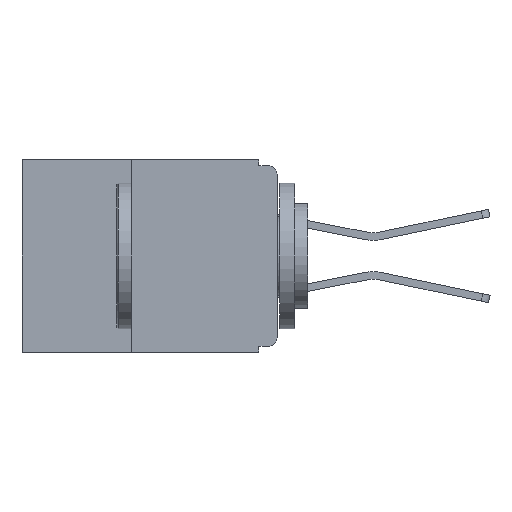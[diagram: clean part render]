
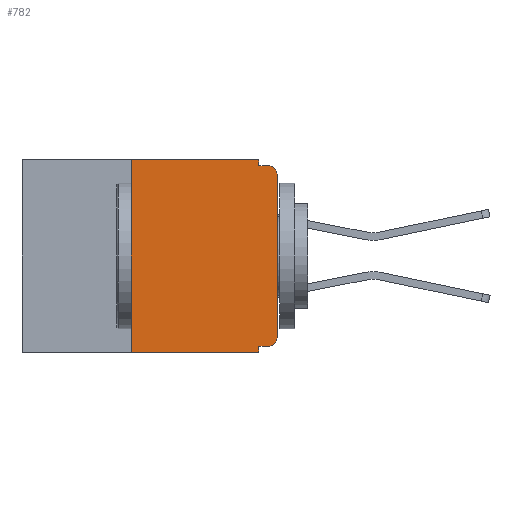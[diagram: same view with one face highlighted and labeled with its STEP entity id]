
A CAD part, left-side view. The second image highlights one B-rep face of the part: STEP entity #782.
In plain terms, the highlighted planar face has unit normal (-1, 0, 0).
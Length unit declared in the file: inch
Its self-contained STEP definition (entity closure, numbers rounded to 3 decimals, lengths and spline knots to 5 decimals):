
#217 = CARTESIAN_POINT ( 'NONE',  ( 0., 0.031, -0.32 ) ) ;
#259 = CARTESIAN_POINT ( 'NONE',  ( 0., 0.031, -0.01 ) ) ;
#279 = FACE_OUTER_BOUND ( 'NONE', #6784, .T. ) ;
#322 = AXIS2_PLACEMENT_3D ( 'NONE', #12585, #4747, #10507 ) ;
#404 = ORIENTED_EDGE ( 'NONE', *, *, #7237, .F. ) ;
#766 = VERTEX_POINT ( 'NONE', #12882 ) ;
#782 = ADVANCED_FACE ( 'NONE', ( #279 ), #10029, .F. ) ;
#824 = VECTOR ( 'NONE', #13183, 39.37008 ) ;
#959 = ORIENTED_EDGE ( 'NONE', *, *, #1504, .F. ) ;
#977 = ORIENTED_EDGE ( 'NONE', *, *, #4737, .F. ) ;
#992 = LINE ( 'NONE', #13202, #824 ) ;
#1199 = VECTOR ( 'NONE', #12674, 39.37008 ) ;
#1253 = LINE ( 'NONE', #12527, #1199 ) ;
#1504 = EDGE_CURVE ( 'NONE', #4203, #4324, #9382, .T. ) ;
#1530 = ORIENTED_EDGE ( 'NONE', *, *, #9431, .F. ) ;
#1769 = CARTESIAN_POINT ( 'NONE',  ( 0., 0.031, -0.33 ) ) ;
#1905 = ORIENTED_EDGE ( 'NONE', *, *, #10928, .T. ) ;
#2468 = VERTEX_POINT ( 'NONE', #11651 ) ;
#3088 = CARTESIAN_POINT ( 'NONE',  ( 0., 0.25, -0.33 ) ) ;
#3165 = CARTESIAN_POINT ( 'NONE',  ( 0., 0.437, 0. ) ) ;
#3212 = VERTEX_POINT ( 'NONE', #11731 ) ;
#3285 = DIRECTION ( 'NONE',  ( 0., -1., 0. ) ) ;
#3527 = DIRECTION ( 'NONE',  ( 0., -1., 0. ) ) ;
#3631 = ORIENTED_EDGE ( 'NONE', *, *, #12496, .F. ) ;
#3725 = CARTESIAN_POINT ( 'NONE',  ( 0., 0.437, -0.33 ) ) ;
#3741 = AXIS2_PLACEMENT_3D ( 'NONE', #12296, #12273, #12238 ) ;
#3754 = DIRECTION ( 'NONE',  ( 0., 0., 1. ) ) ;
#4045 = CARTESIAN_POINT ( 'NONE',  ( 0., 0.25, -0.33 ) ) ;
#4054 = ORIENTED_EDGE ( 'NONE', *, *, #11316, .F. ) ;
#4203 = VERTEX_POINT ( 'NONE', #8209 ) ;
#4324 = VERTEX_POINT ( 'NONE', #259 ) ;
#4660 = ORIENTED_EDGE ( 'NONE', *, *, #10430, .T. ) ;
#4737 = EDGE_CURVE ( 'NONE', #2468, #4203, #6745, .T. ) ;
#4747 = DIRECTION ( 'NONE',  ( 1., 0., 0. ) ) ;
#4825 = VERTEX_POINT ( 'NONE', #217 ) ;
#5218 = VECTOR ( 'NONE', #5842, 39.37008 ) ;
#5301 = VERTEX_POINT ( 'NONE', #12934 ) ;
#5391 = LINE ( 'NONE', #5597, #5218 ) ;
#5597 = CARTESIAN_POINT ( 'NONE',  ( 0., 0., 0. ) ) ;
#5767 = LINE ( 'NONE', #12099, #6563 ) ;
#5842 = DIRECTION ( 'NONE',  ( 0., 0., 1. ) ) ;
#6563 = VECTOR ( 'NONE', #11837, 39.37008 ) ;
#6629 = VERTEX_POINT ( 'NONE', #3088 ) ;
#6683 = VECTOR ( 'NONE', #3285, 39.37008 ) ;
#6727 = VERTEX_POINT ( 'NONE', #1769 ) ;
#6745 = LINE ( 'NONE', #3165, #6683 ) ;
#6784 = EDGE_LOOP ( 'NONE', ( #12923, #12953, #404, #959, #977, #1530, #1905, #3631, #4054, #4660 ) ) ;
#7237 = EDGE_CURVE ( 'NONE', #4324, #11609, #992, .T. ) ;
#7252 = VECTOR ( 'NONE', #3527, 39.37008 ) ;
#7267 = LINE ( 'NONE', #3725, #7252 ) ;
#8209 = CARTESIAN_POINT ( 'NONE',  ( 0., 0.031, 0. ) ) ;
#8455 = EDGE_CURVE ( 'NONE', #5301, #11609, #10012, .T. ) ;
#9232 = CIRCLE ( 'NONE', #12572, 0.015 ) ;
#9303 = VECTOR ( 'NONE', #11578, 39.37008 ) ;
#9382 = LINE ( 'NONE', #12189, #9303 ) ;
#9431 = EDGE_CURVE ( 'NONE', #6629, #2468, #12599, .T. ) ;
#10012 = CIRCLE ( 'NONE', #3741, 0.015 ) ;
#10029 = PLANE ( 'NONE',  #322 ) ;
#10215 = DIRECTION ( 'NONE',  ( 0., 0., -1. ) ) ;
#10248 = DIRECTION ( 'NONE',  ( -1., 0., 0. ) ) ;
#10332 = CARTESIAN_POINT ( 'NONE',  ( 0., 0.015, -0.305 ) ) ;
#10430 = EDGE_CURVE ( 'NONE', #766, #3212, #9232, .T. ) ;
#10507 = DIRECTION ( 'NONE',  ( 0., 0., -1. ) ) ;
#10928 = EDGE_CURVE ( 'NONE', #6629, #6727, #7267, .T. ) ;
#11316 = EDGE_CURVE ( 'NONE', #766, #4825, #5767, .T. ) ;
#11501 = EDGE_CURVE ( 'NONE', #3212, #5301, #5391, .T. ) ;
#11578 = DIRECTION ( 'NONE',  ( 0., 0., -1. ) ) ;
#11609 = VERTEX_POINT ( 'NONE', #12004 ) ;
#11651 = CARTESIAN_POINT ( 'NONE',  ( 0., 0.25, 0. ) ) ;
#11731 = CARTESIAN_POINT ( 'NONE',  ( 0., 0., -0.305 ) ) ;
#11837 = DIRECTION ( 'NONE',  ( 0., 1., 0. ) ) ;
#12004 = CARTESIAN_POINT ( 'NONE',  ( 0., 0.015, -0.01 ) ) ;
#12099 = CARTESIAN_POINT ( 'NONE',  ( 0., 0., -0.32 ) ) ;
#12189 = CARTESIAN_POINT ( 'NONE',  ( 0., 0.031, 0. ) ) ;
#12238 = DIRECTION ( 'NONE',  ( 0., 0., -1. ) ) ;
#12273 = DIRECTION ( 'NONE',  ( -1., 0., 0. ) ) ;
#12296 = CARTESIAN_POINT ( 'NONE',  ( 0., 0.015, -0.025 ) ) ;
#12496 = EDGE_CURVE ( 'NONE', #4825, #6727, #1253, .T. ) ;
#12525 = VECTOR ( 'NONE', #3754, 39.37008 ) ;
#12527 = CARTESIAN_POINT ( 'NONE',  ( 0., 0.031, -0.33 ) ) ;
#12572 = AXIS2_PLACEMENT_3D ( 'NONE', #10332, #10248, #10215 ) ;
#12585 = CARTESIAN_POINT ( 'NONE',  ( 0., 0.437, 0. ) ) ;
#12599 = LINE ( 'NONE', #4045, #12525 ) ;
#12674 = DIRECTION ( 'NONE',  ( 0., 0., -1. ) ) ;
#12882 = CARTESIAN_POINT ( 'NONE',  ( 0., 0.015, -0.32 ) ) ;
#12923 = ORIENTED_EDGE ( 'NONE', *, *, #11501, .T. ) ;
#12934 = CARTESIAN_POINT ( 'NONE',  ( 0., 0., -0.025 ) ) ;
#12953 = ORIENTED_EDGE ( 'NONE', *, *, #8455, .T. ) ;
#13183 = DIRECTION ( 'NONE',  ( 0., -1., 0. ) ) ;
#13202 = CARTESIAN_POINT ( 'NONE',  ( 0., 0., -0.01 ) ) ;
